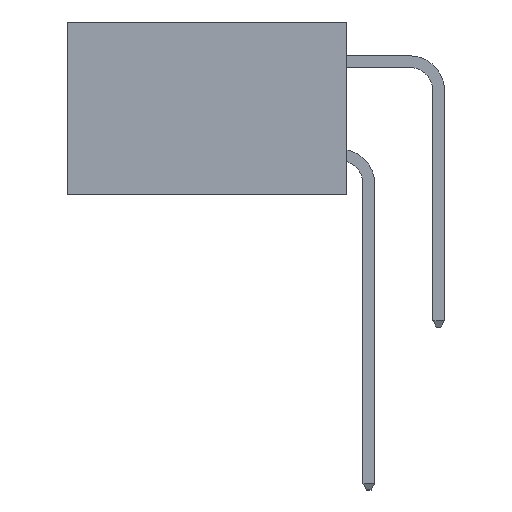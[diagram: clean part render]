
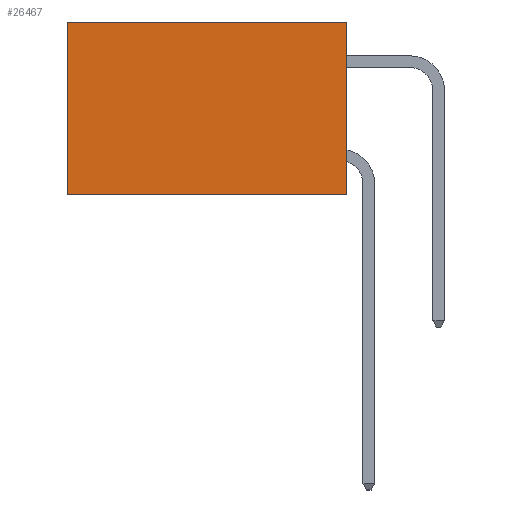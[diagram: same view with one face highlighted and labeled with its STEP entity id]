
A CAD part, left-side view. The second image highlights one B-rep face of the part: STEP entity #26467.
In plain terms, the highlighted planar face has unit normal (-1, 0, 0).
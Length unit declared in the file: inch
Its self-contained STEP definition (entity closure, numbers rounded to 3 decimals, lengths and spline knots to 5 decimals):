
#1390 = VECTOR ( 'NONE', #4230, 39.37008 ) ;
#1704 = EDGE_CURVE ( 'NONE', #9685, #23909, #10520, .T. ) ;
#1718 = ORIENTED_EDGE ( 'NONE', *, *, #1704, .F. ) ;
#1770 = CARTESIAN_POINT ( 'NONE',  ( 0.2875, 0., 0. ) ) ;
#2909 = CARTESIAN_POINT ( 'NONE',  ( 0.2875, 0., 0. ) ) ;
#4230 = DIRECTION ( 'NONE',  ( 0., 0., -1. ) ) ;
#4418 = CARTESIAN_POINT ( 'NONE',  ( 0.2875, 0.6, 0. ) ) ;
#7449 = VERTEX_POINT ( 'NONE', #27458 ) ;
#8820 = CARTESIAN_POINT ( 'NONE',  ( 0.2875, 0., 0. ) ) ;
#9663 = ORIENTED_EDGE ( 'NONE', *, *, #22362, .F. ) ;
#9685 = VERTEX_POINT ( 'NONE', #8820 ) ;
#10520 = LINE ( 'NONE', #1770, #33451 ) ;
#12503 = EDGE_CURVE ( 'NONE', #7449, #33372, #13931, .T. ) ;
#13931 = LINE ( 'NONE', #4418, #1390 ) ;
#14567 = PLANE ( 'NONE',  #23474 ) ;
#14734 = VECTOR ( 'NONE', #24427, 39.37008 ) ;
#15593 = CARTESIAN_POINT ( 'NONE',  ( 0.2875, 0., -0.37 ) ) ;
#16276 = CARTESIAN_POINT ( 'NONE',  ( 0.2875, 0., 0. ) ) ;
#17105 = VECTOR ( 'NONE', #37699, 39.37008 ) ;
#22362 = EDGE_CURVE ( 'NONE', #23909, #33372, #34617, .T. ) ;
#23474 = AXIS2_PLACEMENT_3D ( 'NONE', #2909, #26204, #23880 ) ;
#23880 = DIRECTION ( 'NONE',  ( 0., 0., -1. ) ) ;
#23909 = VERTEX_POINT ( 'NONE', #15593 ) ;
#24427 = DIRECTION ( 'NONE',  ( 0., 1., 0. ) ) ;
#25977 = EDGE_CURVE ( 'NONE', #9685, #7449, #27910, .T. ) ;
#26204 = DIRECTION ( 'NONE',  ( 1., 0., 0. ) ) ;
#26467 = ADVANCED_FACE ( 'NONE', ( #26595 ), #14567, .F. ) ;
#26595 = FACE_OUTER_BOUND ( 'NONE', #29190, .T. ) ;
#27458 = CARTESIAN_POINT ( 'NONE',  ( 0.2875, 0.6, 0. ) ) ;
#27910 = LINE ( 'NONE', #16276, #14734 ) ;
#29190 = EDGE_LOOP ( 'NONE', ( #37623, #9663, #1718, #32336 ) ) ;
#32336 = ORIENTED_EDGE ( 'NONE', *, *, #25977, .T. ) ;
#33372 = VERTEX_POINT ( 'NONE', #34962 ) ;
#33451 = VECTOR ( 'NONE', #37482, 39.37008 ) ;
#34617 = LINE ( 'NONE', #37894, #17105 ) ;
#34962 = CARTESIAN_POINT ( 'NONE',  ( 0.2875, 0.6, -0.37 ) ) ;
#37482 = DIRECTION ( 'NONE',  ( 0., 0., -1. ) ) ;
#37623 = ORIENTED_EDGE ( 'NONE', *, *, #12503, .T. ) ;
#37699 = DIRECTION ( 'NONE',  ( 0., 1., 0. ) ) ;
#37894 = CARTESIAN_POINT ( 'NONE',  ( 0.2875, 0., -0.37 ) ) ;
